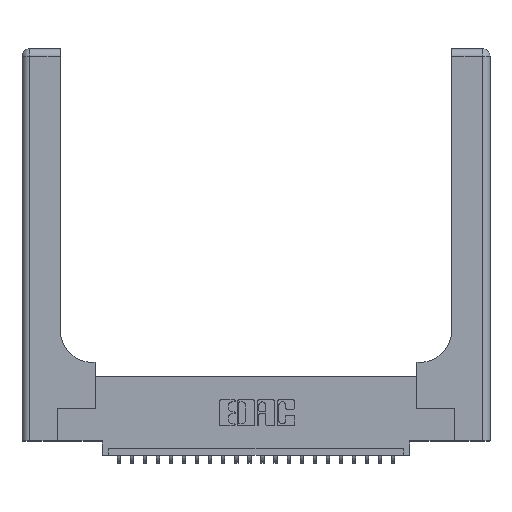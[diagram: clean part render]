
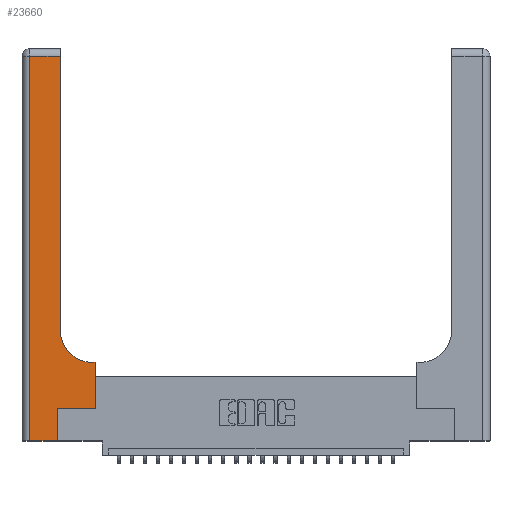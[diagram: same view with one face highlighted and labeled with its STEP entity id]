
A CAD part, top view. The second image highlights one B-rep face of the part: STEP entity #23660.
In plain terms, the highlighted planar face has unit normal (0, 0, 1).
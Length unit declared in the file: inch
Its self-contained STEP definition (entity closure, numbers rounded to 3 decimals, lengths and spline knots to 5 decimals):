
#247 = LINE ( 'NONE', #23206, #11529 ) ;
#264 = VERTEX_POINT ( 'NONE', #12765 ) ;
#1127 = EDGE_CURVE ( 'NONE', #17174, #4465, #10390, .T. ) ;
#1508 = EDGE_CURVE ( 'NONE', #23316, #264, #11865, .T. ) ;
#1515 = VECTOR ( 'NONE', #18810, 39.37008 ) ;
#1657 = CARTESIAN_POINT ( 'NONE',  ( 0.06, 0., 0.37 ) ) ;
#1953 = CARTESIAN_POINT ( 'NONE',  ( 0.2915, 2.94, 0.37 ) ) ;
#2125 = EDGE_CURVE ( 'NONE', #11354, #4833, #9273, .T. ) ;
#2328 = VERTEX_POINT ( 'NONE', #20712 ) ;
#2900 = DIRECTION ( 'NONE',  ( -1., 0., 0. ) ) ;
#3317 = ORIENTED_EDGE ( 'NONE', *, *, #9495, .T. ) ;
#3472 = ORIENTED_EDGE ( 'NONE', *, *, #2125, .T. ) ;
#4465 = VERTEX_POINT ( 'NONE', #14900 ) ;
#4499 = DIRECTION ( 'NONE',  ( -1., 0., 0. ) ) ;
#4535 = CARTESIAN_POINT ( 'NONE',  ( 0.269, 0.25, 0.37 ) ) ;
#4790 = DIRECTION ( 'NONE',  ( 0., 1., 0. ) ) ;
#4833 = VERTEX_POINT ( 'NONE', #1953 ) ;
#4847 = LINE ( 'NONE', #16063, #12610 ) ;
#5460 = ORIENTED_EDGE ( 'NONE', *, *, #1127, .T. ) ;
#5539 = DIRECTION ( 'NONE',  ( 1., 0., 0. ) ) ;
#5856 = DIRECTION ( 'NONE',  ( 0., -1., 0. ) ) ;
#6337 = DIRECTION ( 'NONE',  ( 1., 0., 0. ) ) ;
#6390 = AXIS2_PLACEMENT_3D ( 'NONE', #21523, #16092, #6337 ) ;
#6476 = VECTOR ( 'NONE', #5539, 39.37008 ) ;
#6534 = DIRECTION ( 'NONE',  ( 1., 0., 0. ) ) ;
#7319 = CARTESIAN_POINT ( 'NONE',  ( 0.5585, 0.25, 0.37 ) ) ;
#7980 = EDGE_LOOP ( 'NONE', ( #3472, #21046, #18979, #12660, #3317, #5460, #19197, #17862, #10892 ) ) ;
#7996 = AXIS2_PLACEMENT_3D ( 'NONE', #14011, #21689, #4499 ) ;
#8214 = CARTESIAN_POINT ( 'NONE',  ( 0.2915, 0.6, 0.37 ) ) ;
#8707 = LINE ( 'NONE', #8214, #23614 ) ;
#9273 = LINE ( 'NONE', #16134, #12467 ) ;
#9495 = EDGE_CURVE ( 'NONE', #264, #17174, #18511, .T. ) ;
#10390 = LINE ( 'NONE', #4535, #21133 ) ;
#10892 = ORIENTED_EDGE ( 'NONE', *, *, #23668, .T. ) ;
#10991 = VERTEX_POINT ( 'NONE', #12431 ) ;
#11036 = VECTOR ( 'NONE', #22643, 39.37008 ) ;
#11354 = VERTEX_POINT ( 'NONE', #11486 ) ;
#11486 = CARTESIAN_POINT ( 'NONE',  ( 0.2915, 0.85, 0.37 ) ) ;
#11529 = VECTOR ( 'NONE', #5856, 39.37008 ) ;
#11722 = EDGE_CURVE ( 'NONE', #4465, #2328, #21774, .T. ) ;
#11865 = LINE ( 'NONE', #15054, #6476 ) ;
#12431 = CARTESIAN_POINT ( 'NONE',  ( 0.06, 2.94, 0.37 ) ) ;
#12467 = VECTOR ( 'NONE', #4790, 39.37008 ) ;
#12610 = VECTOR ( 'NONE', #2900, 39.37008 ) ;
#12660 = ORIENTED_EDGE ( 'NONE', *, *, #1508, .T. ) ;
#12765 = CARTESIAN_POINT ( 'NONE',  ( 0.269, 0., 0.37 ) ) ;
#13380 = VERTEX_POINT ( 'NONE', #15348 ) ;
#13594 = EDGE_CURVE ( 'NONE', #4833, #10991, #4847, .T. ) ;
#13810 = FACE_OUTER_BOUND ( 'NONE', #7980, .T. ) ;
#14011 = CARTESIAN_POINT ( 'NONE',  ( 0., 3., 0.37 ) ) ;
#14900 = CARTESIAN_POINT ( 'NONE',  ( 0.5585, 0.25, 0.37 ) ) ;
#14974 = CARTESIAN_POINT ( 'NONE',  ( 0.269, 0., 0.37 ) ) ;
#15054 = CARTESIAN_POINT ( 'NONE',  ( 0., 0., 0.37 ) ) ;
#15348 = CARTESIAN_POINT ( 'NONE',  ( 0.5415, 0.6, 0.37 ) ) ;
#16063 = CARTESIAN_POINT ( 'NONE',  ( 0., 2.94, 0.37 ) ) ;
#16092 = DIRECTION ( 'NONE',  ( 0., 0., -1. ) ) ;
#16134 = CARTESIAN_POINT ( 'NONE',  ( 0.2915, 3., 0.37 ) ) ;
#17174 = VERTEX_POINT ( 'NONE', #21502 ) ;
#17817 = EDGE_CURVE ( 'NONE', #2328, #13380, #8707, .T. ) ;
#17862 = ORIENTED_EDGE ( 'NONE', *, *, #17817, .T. ) ;
#18511 = LINE ( 'NONE', #14974, #11036 ) ;
#18810 = DIRECTION ( 'NONE',  ( 0., 1., 0. ) ) ;
#18979 = ORIENTED_EDGE ( 'NONE', *, *, #20466, .T. ) ;
#19197 = ORIENTED_EDGE ( 'NONE', *, *, #11722, .T. ) ;
#19800 = DIRECTION ( 'NONE',  ( -1., 0., 0. ) ) ;
#20466 = EDGE_CURVE ( 'NONE', #10991, #23316, #247, .T. ) ;
#20712 = CARTESIAN_POINT ( 'NONE',  ( 0.5585, 0.6, 0.37 ) ) ;
#21046 = ORIENTED_EDGE ( 'NONE', *, *, #13594, .T. ) ;
#21133 = VECTOR ( 'NONE', #6534, 39.37008 ) ;
#21502 = CARTESIAN_POINT ( 'NONE',  ( 0.269, 0.25, 0.37 ) ) ;
#21523 = CARTESIAN_POINT ( 'NONE',  ( 0.5415, 0.85, 0.37 ) ) ;
#21689 = DIRECTION ( 'NONE',  ( 0., 0., -1. ) ) ;
#21768 = PLANE ( 'NONE',  #7996 ) ;
#21774 = LINE ( 'NONE', #7319, #1515 ) ;
#22643 = DIRECTION ( 'NONE',  ( 0., 1., 0. ) ) ;
#23206 = CARTESIAN_POINT ( 'NONE',  ( 0.06, 3., 0.37 ) ) ;
#23316 = VERTEX_POINT ( 'NONE', #1657 ) ;
#23614 = VECTOR ( 'NONE', #19800, 39.37008 ) ;
#23660 = ADVANCED_FACE ( 'NONE', ( #13810 ), #21768, .F. ) ;
#23668 = EDGE_CURVE ( 'NONE', #13380, #11354, #24580, .T. ) ;
#24580 = CIRCLE ( 'NONE', #6390, 0.25 ) ;
